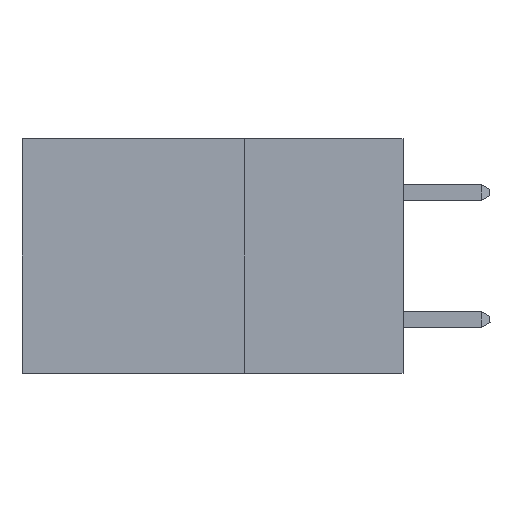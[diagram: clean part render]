
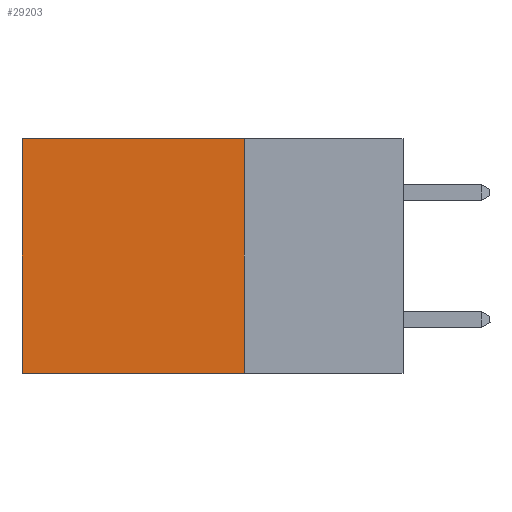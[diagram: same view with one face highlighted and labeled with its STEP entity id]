
A CAD part, left-side view. The second image highlights one B-rep face of the part: STEP entity #29203.
In plain terms, the highlighted planar face has unit normal (-1, 0, 0).
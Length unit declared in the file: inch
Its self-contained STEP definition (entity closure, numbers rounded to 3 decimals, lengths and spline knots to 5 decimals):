
#1185 = ORIENTED_EDGE ( 'NONE', *, *, #35826, .T. ) ;
#1880 = DIRECTION ( 'NONE',  ( 0., 0., -1. ) ) ;
#2669 = CARTESIAN_POINT ( 'NONE',  ( 0.2875, 0.25, 0. ) ) ;
#2863 = VECTOR ( 'NONE', #33777, 39.37008 ) ;
#3869 = AXIS2_PLACEMENT_3D ( 'NONE', #17129, #38801, #1880 ) ;
#4462 = VECTOR ( 'NONE', #31535, 39.37008 ) ;
#5143 = CARTESIAN_POINT ( 'NONE',  ( 0.2875, 0.25, 0. ) ) ;
#8913 = FACE_OUTER_BOUND ( 'NONE', #9464, .T. ) ;
#9464 = EDGE_LOOP ( 'NONE', ( #1185, #15553, #32279, #16828 ) ) ;
#10682 = LINE ( 'NONE', #5143, #26908 ) ;
#11927 = VERTEX_POINT ( 'NONE', #12268 ) ;
#11995 = VERTEX_POINT ( 'NONE', #28403 ) ;
#12268 = CARTESIAN_POINT ( 'NONE',  ( 0.2875, 0.6, 0. ) ) ;
#12603 = LINE ( 'NONE', #15982, #4462 ) ;
#15553 = ORIENTED_EDGE ( 'NONE', *, *, #24671, .F. ) ;
#15982 = CARTESIAN_POINT ( 'NONE',  ( 0.2875, 0.25, -0.37 ) ) ;
#16553 = LINE ( 'NONE', #26702, #23670 ) ;
#16701 = CARTESIAN_POINT ( 'NONE',  ( 0.2875, 0.6, -0.37 ) ) ;
#16828 = ORIENTED_EDGE ( 'NONE', *, *, #21081, .T. ) ;
#17129 = CARTESIAN_POINT ( 'NONE',  ( 0.2875, 0.25, 0. ) ) ;
#17952 = VERTEX_POINT ( 'NONE', #2669 ) ;
#19132 = LINE ( 'NONE', #28724, #2863 ) ;
#21081 = EDGE_CURVE ( 'NONE', #17952, #11927, #16553, .T. ) ;
#23670 = VECTOR ( 'NONE', #36404, 39.37008 ) ;
#24671 = EDGE_CURVE ( 'NONE', #11995, #32597, #12603, .T. ) ;
#24970 = DIRECTION ( 'NONE',  ( 0., 0., -1. ) ) ;
#26702 = CARTESIAN_POINT ( 'NONE',  ( 0.2875, 0.25, 0. ) ) ;
#26908 = VECTOR ( 'NONE', #24970, 39.37008 ) ;
#28403 = CARTESIAN_POINT ( 'NONE',  ( 0.2875, 0.25, -0.37 ) ) ;
#28724 = CARTESIAN_POINT ( 'NONE',  ( 0.2875, 0.6, 0. ) ) ;
#29203 = ADVANCED_FACE ( 'NONE', ( #8913 ), #32299, .F. ) ;
#31535 = DIRECTION ( 'NONE',  ( 0., 1., 0. ) ) ;
#32279 = ORIENTED_EDGE ( 'NONE', *, *, #33535, .F. ) ;
#32299 = PLANE ( 'NONE',  #3869 ) ;
#32597 = VERTEX_POINT ( 'NONE', #16701 ) ;
#33535 = EDGE_CURVE ( 'NONE', #17952, #11995, #10682, .T. ) ;
#33777 = DIRECTION ( 'NONE',  ( 0., 0., -1. ) ) ;
#35826 = EDGE_CURVE ( 'NONE', #11927, #32597, #19132, .T. ) ;
#36404 = DIRECTION ( 'NONE',  ( 0., 1., 0. ) ) ;
#38801 = DIRECTION ( 'NONE',  ( 1., 0., 0. ) ) ;
